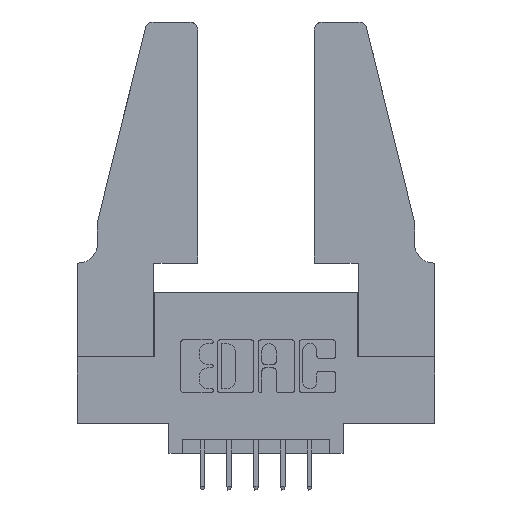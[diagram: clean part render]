
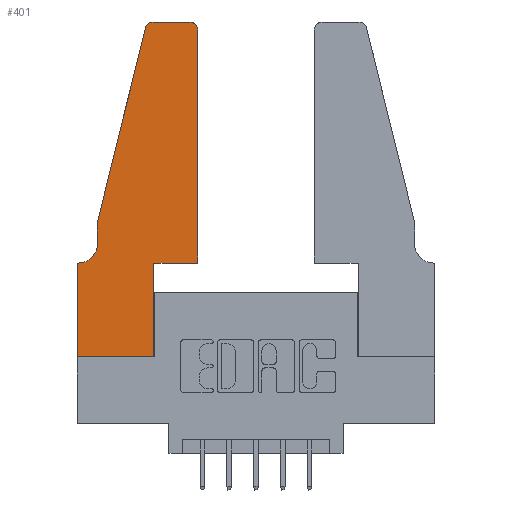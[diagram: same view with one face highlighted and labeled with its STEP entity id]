
A CAD part, top view. The second image highlights one B-rep face of the part: STEP entity #401.
In plain terms, the highlighted planar face has unit normal (0, 0, 1).
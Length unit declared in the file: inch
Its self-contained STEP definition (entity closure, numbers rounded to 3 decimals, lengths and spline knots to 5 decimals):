
#59 = EDGE_CURVE ( 'NONE', #2348, #9959, #1750, .T. ) ;
#292 = ORIENTED_EDGE ( 'NONE', *, *, #662, .T. ) ;
#351 = LINE ( 'NONE', #4730, #2235 ) ;
#379 = VECTOR ( 'NONE', #10327, 39.37008 ) ;
#401 = ADVANCED_FACE ( 'NONE', ( #10589 ), #9514, .T. ) ;
#432 = VECTOR ( 'NONE', #11274, 39.37008 ) ;
#440 = DIRECTION ( 'NONE',  ( 0., 0., 1. ) ) ;
#510 = CARTESIAN_POINT ( 'NONE',  ( 0.2865, 0.35, 0.37 ) ) ;
#662 = EDGE_CURVE ( 'NONE', #5517, #1547, #6922, .T. ) ;
#914 = DIRECTION ( 'NONE',  ( 0., 0., 1. ) ) ;
#962 = EDGE_CURVE ( 'NONE', #5739, #4776, #7904, .T. ) ;
#1043 = EDGE_CURVE ( 'NONE', #2602, #9321, #11052, .T. ) ;
#1156 = VECTOR ( 'NONE', #6813, 39.37008 ) ;
#1178 = ORIENTED_EDGE ( 'NONE', *, *, #1043, .T. ) ;
#1210 = ORIENTED_EDGE ( 'NONE', *, *, #7989, .T. ) ;
#1245 = ORIENTED_EDGE ( 'NONE', *, *, #1706, .T. ) ;
#1433 = LINE ( 'NONE', #6664, #7645 ) ;
#1515 = CARTESIAN_POINT ( 'NONE',  ( 0., 0.35, 0.37 ) ) ;
#1547 = VERTEX_POINT ( 'NONE', #2806 ) ;
#1607 = EDGE_LOOP ( 'NONE', ( #5151, #9838, #10377, #3432, #1210, #6009, #1178, #10868, #5670, #292, #1245, #4048 ) ) ;
#1706 = EDGE_CURVE ( 'NONE', #1547, #7477, #351, .T. ) ;
#1750 = LINE ( 'NONE', #7767, #432 ) ;
#1920 = LINE ( 'NONE', #7073, #7717 ) ;
#1934 = DIRECTION ( 'NONE',  ( 1., 0., 0. ) ) ;
#2023 = DIRECTION ( 'NONE',  ( -0.239, -0.971, 0. ) ) ;
#2235 = VECTOR ( 'NONE', #2915, 39.37008 ) ;
#2239 = CARTESIAN_POINT ( 'NONE',  ( 0., 0., 0.37 ) ) ;
#2334 = EDGE_CURVE ( 'NONE', #3238, #5517, #8320, .T. ) ;
#2348 = VERTEX_POINT ( 'NONE', #2871 ) ;
#2409 = EDGE_CURVE ( 'NONE', #4535, #5739, #9475, .T. ) ;
#2562 = CARTESIAN_POINT ( 'NONE',  ( 0.0055, 0.42, 0.37 ) ) ;
#2602 = VERTEX_POINT ( 'NONE', #1515 ) ;
#2806 = CARTESIAN_POINT ( 'NONE',  ( 0.4505, 0.35, 0.37 ) ) ;
#2871 = CARTESIAN_POINT ( 'NONE',  ( 0.0755, 0.5, 0.37 ) ) ;
#2915 = DIRECTION ( 'NONE',  ( 0., 1., 0. ) ) ;
#3040 = CARTESIAN_POINT ( 'NONE',  ( 0.4205, 1.25, 0.37 ) ) ;
#3124 = DIRECTION ( 'NONE',  ( 0., 1., 0. ) ) ;
#3172 = AXIS2_PLACEMENT_3D ( 'NONE', #10777, #440, #9931 ) ;
#3212 = EDGE_CURVE ( 'NONE', #7477, #4535, #8972, .T. ) ;
#3238 = VERTEX_POINT ( 'NONE', #6209 ) ;
#3432 = ORIENTED_EDGE ( 'NONE', *, *, #59, .T. ) ;
#3467 = CARTESIAN_POINT ( 'NONE',  ( 0.4205, 1.22, 0.37 ) ) ;
#4048 = ORIENTED_EDGE ( 'NONE', *, *, #3212, .T. ) ;
#4286 = CARTESIAN_POINT ( 'NONE',  ( 0., 0.35, 0.37 ) ) ;
#4535 = VERTEX_POINT ( 'NONE', #3040 ) ;
#4730 = CARTESIAN_POINT ( 'NONE',  ( 0.4505, 0.35, 0.37 ) ) ;
#4776 = VERTEX_POINT ( 'NONE', #6606 ) ;
#5151 = ORIENTED_EDGE ( 'NONE', *, *, #2409, .T. ) ;
#5368 = CARTESIAN_POINT ( 'NONE',  ( 0.2605, 1.25, 0.37 ) ) ;
#5418 = EDGE_CURVE ( 'NONE', #10570, #2602, #6075, .T. ) ;
#5517 = VERTEX_POINT ( 'NONE', #9978 ) ;
#5670 = ORIENTED_EDGE ( 'NONE', *, *, #2334, .T. ) ;
#5739 = VERTEX_POINT ( 'NONE', #8353 ) ;
#5773 = DIRECTION ( 'NONE',  ( 0., -1., 0. ) ) ;
#6000 = CARTESIAN_POINT ( 'NONE',  ( 0., 0., 0.37 ) ) ;
#6009 = ORIENTED_EDGE ( 'NONE', *, *, #5418, .T. ) ;
#6041 = EDGE_CURVE ( 'NONE', #4776, #2348, #1920, .T. ) ;
#6075 = LINE ( 'NONE', #10318, #11196 ) ;
#6209 = CARTESIAN_POINT ( 'NONE',  ( 0.2865, 0., 0.37 ) ) ;
#6606 = CARTESIAN_POINT ( 'NONE',  ( 0.25487, 1.22718, 0.37 ) ) ;
#6664 = CARTESIAN_POINT ( 'NONE',  ( 0., 0., 0.37 ) ) ;
#6813 = DIRECTION ( 'NONE',  ( 1., 0., 0. ) ) ;
#6922 = LINE ( 'NONE', #8540, #1156 ) ;
#7073 = CARTESIAN_POINT ( 'NONE',  ( 0.0755, 0.5, 0.37 ) ) ;
#7477 = VERTEX_POINT ( 'NONE', #10874 ) ;
#7645 = VECTOR ( 'NONE', #10224, 39.37008 ) ;
#7717 = VECTOR ( 'NONE', #2023, 39.37008 ) ;
#7745 = DIRECTION ( 'NONE',  ( 0., 0., -1. ) ) ;
#7767 = CARTESIAN_POINT ( 'NONE',  ( 0.0755, 0.5, 0.37 ) ) ;
#7871 = DIRECTION ( 'NONE',  ( 1., 0., 0. ) ) ;
#7904 = CIRCLE ( 'NONE', #3172, 0.03 ) ;
#7989 = EDGE_CURVE ( 'NONE', #9959, #10570, #9686, .T. ) ;
#8082 = AXIS2_PLACEMENT_3D ( 'NONE', #4286, #10426, #1934 ) ;
#8320 = LINE ( 'NONE', #510, #10632 ) ;
#8353 = CARTESIAN_POINT ( 'NONE',  ( 0.284, 1.25, 0.37 ) ) ;
#8540 = CARTESIAN_POINT ( 'NONE',  ( 0.4505, 0.35, 0.37 ) ) ;
#8551 = DIRECTION ( 'NONE',  ( -1., 0., 0. ) ) ;
#8972 = CIRCLE ( 'NONE', #9165, 0.03 ) ;
#9165 = AXIS2_PLACEMENT_3D ( 'NONE', #3467, #914, #7871 ) ;
#9265 = EDGE_CURVE ( 'NONE', #9321, #3238, #1433, .T. ) ;
#9321 = VERTEX_POINT ( 'NONE', #2239 ) ;
#9475 = LINE ( 'NONE', #5368, #379 ) ;
#9514 = PLANE ( 'NONE',  #8082 ) ;
#9593 = DIRECTION ( 'NONE',  ( -1., 0., 0. ) ) ;
#9686 = CIRCLE ( 'NONE', #11121, 0.07 ) ;
#9838 = ORIENTED_EDGE ( 'NONE', *, *, #962, .T. ) ;
#9931 = DIRECTION ( 'NONE',  ( 1., 0., 0. ) ) ;
#9959 = VERTEX_POINT ( 'NONE', #10028 ) ;
#9978 = CARTESIAN_POINT ( 'NONE',  ( 0.2865, 0.35, 0.37 ) ) ;
#10028 = CARTESIAN_POINT ( 'NONE',  ( 0.0755, 0.42, 0.37 ) ) ;
#10180 = CARTESIAN_POINT ( 'NONE',  ( 0.0055, 0.35, 0.37 ) ) ;
#10224 = DIRECTION ( 'NONE',  ( 1., 0., 0. ) ) ;
#10318 = CARTESIAN_POINT ( 'NONE',  ( 0.0755, 0.35, 0.37 ) ) ;
#10327 = DIRECTION ( 'NONE',  ( -1., 0., 0. ) ) ;
#10377 = ORIENTED_EDGE ( 'NONE', *, *, #6041, .T. ) ;
#10426 = DIRECTION ( 'NONE',  ( 0., 0., 1. ) ) ;
#10491 = VECTOR ( 'NONE', #5773, 39.37008 ) ;
#10570 = VERTEX_POINT ( 'NONE', #10180 ) ;
#10589 = FACE_OUTER_BOUND ( 'NONE', #1607, .T. ) ;
#10632 = VECTOR ( 'NONE', #3124, 39.37008 ) ;
#10777 = CARTESIAN_POINT ( 'NONE',  ( 0.284, 1.22, 0.37 ) ) ;
#10868 = ORIENTED_EDGE ( 'NONE', *, *, #9265, .T. ) ;
#10874 = CARTESIAN_POINT ( 'NONE',  ( 0.4505, 1.22, 0.37 ) ) ;
#11052 = LINE ( 'NONE', #6000, #10491 ) ;
#11121 = AXIS2_PLACEMENT_3D ( 'NONE', #2562, #7745, #8551 ) ;
#11196 = VECTOR ( 'NONE', #9593, 39.37008 ) ;
#11274 = DIRECTION ( 'NONE',  ( 0., -1., 0. ) ) ;
